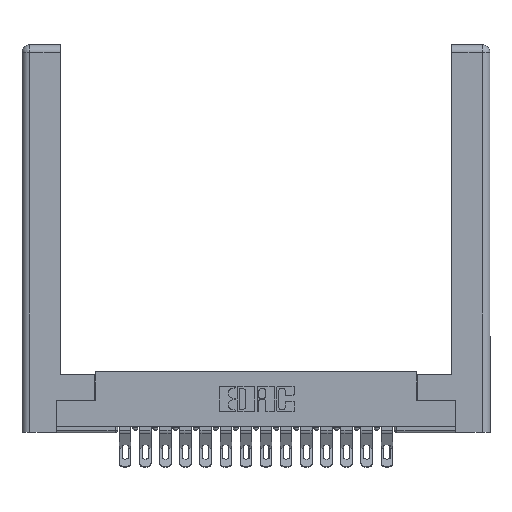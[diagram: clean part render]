
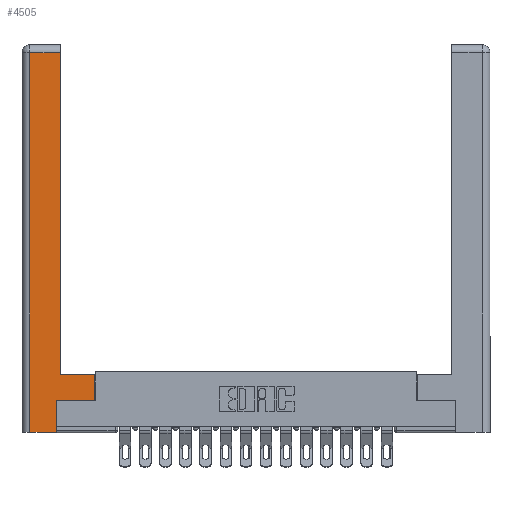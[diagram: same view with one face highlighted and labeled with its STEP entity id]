
A CAD part, top view. The second image highlights one B-rep face of the part: STEP entity #4505.
In plain terms, the highlighted planar face has unit normal (0, 0, 1).
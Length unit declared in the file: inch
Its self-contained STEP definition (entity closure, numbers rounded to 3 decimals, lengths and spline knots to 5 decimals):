
#106 = CARTESIAN_POINT ( 'NONE',  ( 0.295, 0.45, 0. ) ) ;
#136 = EDGE_CURVE ( 'NONE', #3195, #11627, #10978, .T. ) ;
#364 = VECTOR ( 'NONE', #6074, 39.37008 ) ;
#695 = DIRECTION ( 'NONE',  ( 0., 1., 0. ) ) ;
#772 = CARTESIAN_POINT ( 'NONE',  ( 0.295, 0.45, 0. ) ) ;
#849 = ORIENTED_EDGE ( 'NONE', *, *, #15357, .T. ) ;
#1186 = VERTEX_POINT ( 'NONE', #6929 ) ;
#1443 = ORIENTED_EDGE ( 'NONE', *, *, #16616, .T. ) ;
#1777 = LINE ( 'NONE', #16382, #6666 ) ;
#1962 = EDGE_LOOP ( 'NONE', ( #13856, #1443, #9877, #8047, #17633, #849, #4765, #5537 ) ) ;
#2142 = VECTOR ( 'NONE', #11054, 39.37008 ) ;
#2240 = CARTESIAN_POINT ( 'NONE',  ( 0.0615, 2.94, 0. ) ) ;
#2434 = VECTOR ( 'NONE', #15769, 39.37008 ) ;
#2548 = CARTESIAN_POINT ( 'NONE',  ( 0.0615, 0., 0. ) ) ;
#3038 = CARTESIAN_POINT ( 'NONE',  ( 0.265, 0.245, 0. ) ) ;
#3195 = VERTEX_POINT ( 'NONE', #2240 ) ;
#4505 = ADVANCED_FACE ( 'NONE', ( #14237 ), #8832, .F. ) ;
#4765 = ORIENTED_EDGE ( 'NONE', *, *, #17994, .T. ) ;
#5073 = CARTESIAN_POINT ( 'NONE',  ( 0.0615, 0., 0. ) ) ;
#5537 = ORIENTED_EDGE ( 'NONE', *, *, #12764, .T. ) ;
#5954 = VERTEX_POINT ( 'NONE', #9531 ) ;
#6032 = CARTESIAN_POINT ( 'NONE',  ( 0., 0., 0. ) ) ;
#6074 = DIRECTION ( 'NONE',  ( 0., 1., 0. ) ) ;
#6666 = VECTOR ( 'NONE', #17837, 39.37008 ) ;
#6929 = CARTESIAN_POINT ( 'NONE',  ( 0.265, 0.245, 0. ) ) ;
#7129 = VERTEX_POINT ( 'NONE', #772 ) ;
#7508 = VECTOR ( 'NONE', #14863, 39.37008 ) ;
#7584 = CARTESIAN_POINT ( 'NONE',  ( 0.265, 0., 0. ) ) ;
#8047 = ORIENTED_EDGE ( 'NONE', *, *, #18787, .T. ) ;
#8293 = VERTEX_POINT ( 'NONE', #7584 ) ;
#8430 = VECTOR ( 'NONE', #695, 39.37008 ) ;
#8600 = CARTESIAN_POINT ( 'NONE',  ( 0.565, 0.245, 0. ) ) ;
#8832 = PLANE ( 'NONE',  #11949 ) ;
#9531 = CARTESIAN_POINT ( 'NONE',  ( 0.565, 0.45, 0. ) ) ;
#9758 = VECTOR ( 'NONE', #13193, 39.37008 ) ;
#9877 = ORIENTED_EDGE ( 'NONE', *, *, #136, .T. ) ;
#10473 = LINE ( 'NONE', #15404, #8430 ) ;
#10672 = EDGE_CURVE ( 'NONE', #8293, #1186, #15814, .T. ) ;
#10978 = LINE ( 'NONE', #2548, #2434 ) ;
#11054 = DIRECTION ( 'NONE',  ( 1., 0., 0. ) ) ;
#11446 = LINE ( 'NONE', #17920, #7508 ) ;
#11581 = LINE ( 'NONE', #17862, #14738 ) ;
#11627 = VERTEX_POINT ( 'NONE', #5073 ) ;
#11949 = AXIS2_PLACEMENT_3D ( 'NONE', #6032, #17780, #13154 ) ;
#12233 = VERTEX_POINT ( 'NONE', #14275 ) ;
#12764 = EDGE_CURVE ( 'NONE', #5954, #7129, #13170, .T. ) ;
#13154 = DIRECTION ( 'NONE',  ( -1., 0., 0. ) ) ;
#13170 = LINE ( 'NONE', #106, #9758 ) ;
#13193 = DIRECTION ( 'NONE',  ( -1., 0., 0. ) ) ;
#13375 = VERTEX_POINT ( 'NONE', #8600 ) ;
#13438 = EDGE_CURVE ( 'NONE', #7129, #12233, #11581, .T. ) ;
#13856 = ORIENTED_EDGE ( 'NONE', *, *, #13438, .T. ) ;
#14237 = FACE_OUTER_BOUND ( 'NONE', #1962, .T. ) ;
#14275 = CARTESIAN_POINT ( 'NONE',  ( 0.295, 2.94, 0. ) ) ;
#14317 = LINE ( 'NONE', #16777, #2142 ) ;
#14738 = VECTOR ( 'NONE', #17612, 39.37008 ) ;
#14863 = DIRECTION ( 'NONE',  ( -1., 0., 0. ) ) ;
#15357 = EDGE_CURVE ( 'NONE', #1186, #13375, #1777, .T. ) ;
#15404 = CARTESIAN_POINT ( 'NONE',  ( 0.565, 0.45, 0. ) ) ;
#15769 = DIRECTION ( 'NONE',  ( 0., -1., 0. ) ) ;
#15814 = LINE ( 'NONE', #3038, #364 ) ;
#16382 = CARTESIAN_POINT ( 'NONE',  ( 0.565, 0.245, 0. ) ) ;
#16616 = EDGE_CURVE ( 'NONE', #12233, #3195, #11446, .T. ) ;
#16777 = CARTESIAN_POINT ( 'NONE',  ( 0.265, 0., 0. ) ) ;
#17612 = DIRECTION ( 'NONE',  ( 0., 1., 0. ) ) ;
#17633 = ORIENTED_EDGE ( 'NONE', *, *, #10672, .T. ) ;
#17780 = DIRECTION ( 'NONE',  ( 0., 0., -1. ) ) ;
#17837 = DIRECTION ( 'NONE',  ( 1., 0., 0. ) ) ;
#17862 = CARTESIAN_POINT ( 'NONE',  ( 0.295, 3., 0. ) ) ;
#17920 = CARTESIAN_POINT ( 'NONE',  ( 0.0615, 2.94, 0. ) ) ;
#17994 = EDGE_CURVE ( 'NONE', #13375, #5954, #10473, .T. ) ;
#18787 = EDGE_CURVE ( 'NONE', #11627, #8293, #14317, .T. ) ;
